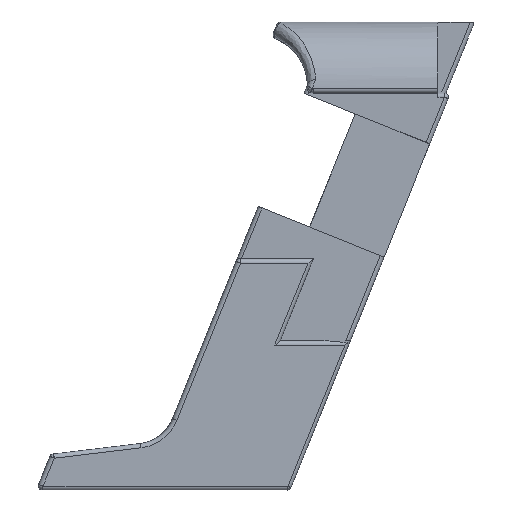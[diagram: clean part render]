
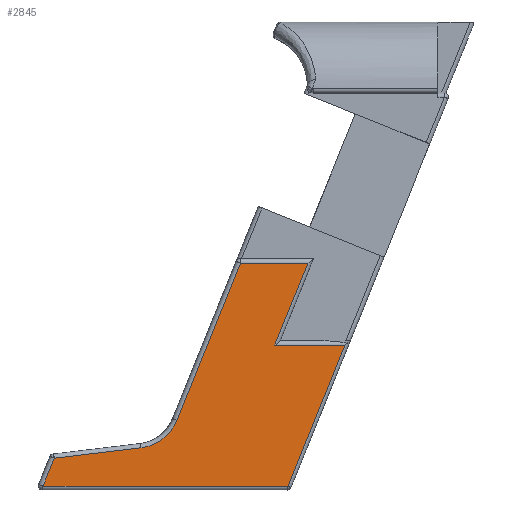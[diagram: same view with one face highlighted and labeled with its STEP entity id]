
A CAD part, left-side view. The second image highlights one B-rep face of the part: STEP entity #2845.
In plain terms, the highlighted planar face has unit normal (-0.989, -0.139, -0.056).
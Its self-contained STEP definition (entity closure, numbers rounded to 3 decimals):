
#333=FACE_OUTER_BOUND('',#508,.T.);
#508=EDGE_LOOP('',(#2403,#2404,#2405,#2406,#2407,#2408,#2409,#2410,#2411));
#730=ELLIPSE('',#3115,2.826,2.794);
#867=LINE('',#5337,#1035);
#868=LINE('',#5340,#1036);
#870=LINE('',#5377,#1038);
#871=LINE('',#5381,#1039);
#874=LINE('',#5390,#1042);
#882=LINE('',#5410,#1050);
#893=LINE('',#5884,#1061);
#894=LINE('',#5885,#1062);
#1035=VECTOR('',#3761,10.);
#1036=VECTOR('',#3764,10.);
#1038=VECTOR('',#3778,10.);
#1039=VECTOR('',#3783,10.);
#1042=VECTOR('',#3792,10.);
#1050=VECTOR('',#3812,10.);
#1061=VECTOR('',#3899,10.);
#1062=VECTOR('',#3900,10.);
#1241=VERTEX_POINT('',#4949);
#1243=VERTEX_POINT('',#4955);
#1251=VERTEX_POINT('',#5086);
#1275=VERTEX_POINT('',#5339);
#1276=VERTEX_POINT('',#5367);
#1279=VERTEX_POINT('',#5376);
#1280=VERTEX_POINT('',#5380);
#1283=VERTEX_POINT('',#5388);
#1312=VERTEX_POINT('',#5883);
#1628=EDGE_CURVE('',#1243,#1241,#867,.T.);
#1629=EDGE_CURVE('',#1241,#1275,#868,.T.);
#1631=EDGE_CURVE('',#1275,#1276,#730,.T.);
#1636=EDGE_CURVE('',#1251,#1279,#870,.T.);
#1638=EDGE_CURVE('',#1280,#1279,#871,.T.);
#1643=EDGE_CURVE('',#1283,#1243,#874,.T.);
#1653=EDGE_CURVE('',#1276,#1251,#882,.T.);
#1699=EDGE_CURVE('',#1312,#1283,#893,.T.);
#1700=EDGE_CURVE('',#1280,#1312,#894,.T.);
#2403=ORIENTED_EDGE('',*,*,#1636,.F.);
#2404=ORIENTED_EDGE('',*,*,#1653,.F.);
#2405=ORIENTED_EDGE('',*,*,#1631,.F.);
#2406=ORIENTED_EDGE('',*,*,#1629,.F.);
#2407=ORIENTED_EDGE('',*,*,#1628,.F.);
#2408=ORIENTED_EDGE('',*,*,#1643,.F.);
#2409=ORIENTED_EDGE('',*,*,#1699,.F.);
#2410=ORIENTED_EDGE('',*,*,#1700,.F.);
#2411=ORIENTED_EDGE('',*,*,#1638,.T.);
#2707=PLANE('',#3168);
#2845=ADVANCED_FACE('',(#333),#2707,.T.);
#3115=AXIS2_PLACEMENT_3D('',#5368,#3767,#3768);
#3168=AXIS2_PLACEMENT_3D('',#5882,#3897,#3898);
#3761=DIRECTION('',(0.,-0.375,0.927));
#3764=DIRECTION('',(0.131,-0.984,0.118));
#3767=DIRECTION('center_axis',(-0.989,-0.139,-0.056));
#3768=DIRECTION('ref_axis',(0.149,-0.917,-0.37));
#3778=DIRECTION('',(0.139,-0.99,0.));
#3783=DIRECTION('',(0.,-0.375,0.927));
#3792=DIRECTION('',(-0.139,0.99,0.));
#3812=DIRECTION('',(0.,-0.375,0.927));
#3897=DIRECTION('center_axis',(-0.989,-0.139,-0.056));
#3898=DIRECTION('ref_axis',(0.149,-0.917,-0.37));
#3899=DIRECTION('',(0.,0.375,-0.927));
#3900=DIRECTION('',(0.139,-0.99,0.));
#4949=CARTESIAN_POINT('',(-12.963,7.744,0.83));
#4955=CARTESIAN_POINT('',(-12.963,8.456,-0.932));
#5086=CARTESIAN_POINT('',(-12.015,-3.979,13.114));
#5337=CARTESIAN_POINT('',(-12.963,7.276,1.987));
#5339=CARTESIAN_POINT('',(-12.234,2.282,1.482));
#5340=CARTESIAN_POINT('',(-13.162,9.236,0.652));
#5367=CARTESIAN_POINT('',(-12.015,0.023,3.21));
#5368=CARTESIAN_POINT('Origin',(-12.438,2.613,4.257));
#5376=CARTESIAN_POINT('',(-11.42,-8.225,13.114));
#5377=CARTESIAN_POINT('',(-12.92,2.476,13.114));
#5380=CARTESIAN_POINT('',(-11.42,-6.141,7.957));
#5381=CARTESIAN_POINT('',(-11.42,-5.413,6.154));
#5388=CARTESIAN_POINT('',(-10.802,-6.96,-0.932));
#5390=CARTESIAN_POINT('',(-12.487,5.064,-0.932));
#5410=CARTESIAN_POINT('',(-12.015,-1.024,5.802));
#5882=CARTESIAN_POINT('Origin',(-13.284,9.621,1.864));
#5883=CARTESIAN_POINT('',(-10.802,-10.552,7.957));
#5884=CARTESIAN_POINT('',(-10.802,-8.466,2.795));
#5885=CARTESIAN_POINT('',(-12.492,1.504,7.957));
